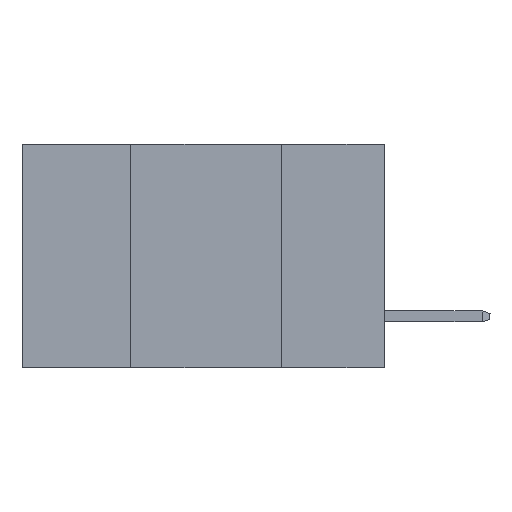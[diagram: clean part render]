
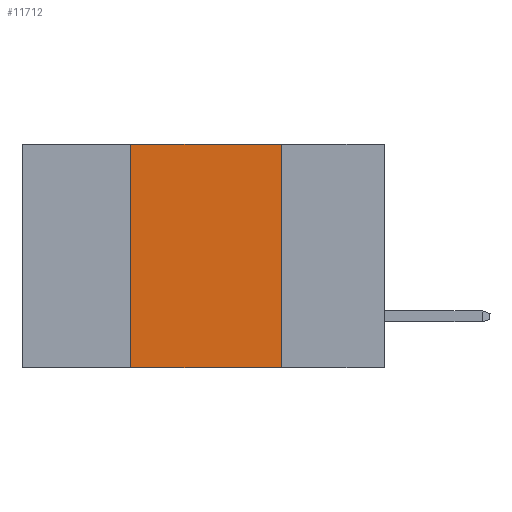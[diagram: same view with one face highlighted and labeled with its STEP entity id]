
A CAD part, left-side view. The second image highlights one B-rep face of the part: STEP entity #11712.
In plain terms, the highlighted planar face has unit normal (-1, 0, 0).
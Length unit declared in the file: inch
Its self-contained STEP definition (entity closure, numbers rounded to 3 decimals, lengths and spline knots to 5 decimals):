
#132 = EDGE_CURVE ( 'NONE', #18474, #2522, #17629, .T. ) ;
#1000 = DIRECTION ( 'NONE',  ( 0., -1., 0. ) ) ;
#1515 = CARTESIAN_POINT ( 'NONE',  ( 0., 0.6, 0. ) ) ;
#1762 = CARTESIAN_POINT ( 'NONE',  ( 0., 0.42, -0.37 ) ) ;
#2349 = CARTESIAN_POINT ( 'NONE',  ( 0., 0.17, -0.37 ) ) ;
#2522 = VERTEX_POINT ( 'NONE', #10041 ) ;
#3239 = ORIENTED_EDGE ( 'NONE', *, *, #11988, .T. ) ;
#3683 = CARTESIAN_POINT ( 'NONE',  ( 0., 0.42, 0. ) ) ;
#3943 = LINE ( 'NONE', #5517, #18125 ) ;
#4598 = CARTESIAN_POINT ( 'NONE',  ( 0., 0.6, 0. ) ) ;
#5178 = CARTESIAN_POINT ( 'NONE',  ( 0., 0.42, -0.37 ) ) ;
#5517 = CARTESIAN_POINT ( 'NONE',  ( 0., 0.6, -0.37 ) ) ;
#5769 = VERTEX_POINT ( 'NONE', #2349 ) ;
#6518 = VECTOR ( 'NONE', #15834, 39.37008 ) ;
#6575 = DIRECTION ( 'NONE',  ( 0., 0., 1. ) ) ;
#7214 = EDGE_CURVE ( 'NONE', #18093, #18474, #10773, .T. ) ;
#8418 = VECTOR ( 'NONE', #13304, 39.37008 ) ;
#8685 = DIRECTION ( 'NONE',  ( 1., 0., 0. ) ) ;
#8879 = DIRECTION ( 'NONE',  ( 0., 0., -1. ) ) ;
#9541 = VECTOR ( 'NONE', #6575, 39.37008 ) ;
#9715 = ORIENTED_EDGE ( 'NONE', *, *, #7214, .F. ) ;
#10041 = CARTESIAN_POINT ( 'NONE',  ( 0., 0.17, 0. ) ) ;
#10773 = LINE ( 'NONE', #1762, #9541 ) ;
#11231 = LINE ( 'NONE', #13965, #6518 ) ;
#11712 = ADVANCED_FACE ( 'NONE', ( #16510 ), #17785, .F. ) ;
#11988 = EDGE_CURVE ( 'NONE', #18093, #5769, #3943, .T. ) ;
#13304 = DIRECTION ( 'NONE',  ( 0., -1., 0. ) ) ;
#13965 = CARTESIAN_POINT ( 'NONE',  ( 0., 0.17, -0.37 ) ) ;
#14568 = EDGE_LOOP ( 'NONE', ( #14824, #18568, #9715, #3239 ) ) ;
#14824 = ORIENTED_EDGE ( 'NONE', *, *, #18484, .F. ) ;
#15306 = AXIS2_PLACEMENT_3D ( 'NONE', #1515, #8685, #8879 ) ;
#15834 = DIRECTION ( 'NONE',  ( 0., 0., -1. ) ) ;
#16510 = FACE_OUTER_BOUND ( 'NONE', #14568, .T. ) ;
#17629 = LINE ( 'NONE', #4598, #8418 ) ;
#17785 = PLANE ( 'NONE',  #15306 ) ;
#18093 = VERTEX_POINT ( 'NONE', #5178 ) ;
#18125 = VECTOR ( 'NONE', #1000, 39.37008 ) ;
#18474 = VERTEX_POINT ( 'NONE', #3683 ) ;
#18484 = EDGE_CURVE ( 'NONE', #2522, #5769, #11231, .T. ) ;
#18568 = ORIENTED_EDGE ( 'NONE', *, *, #132, .F. ) ;
